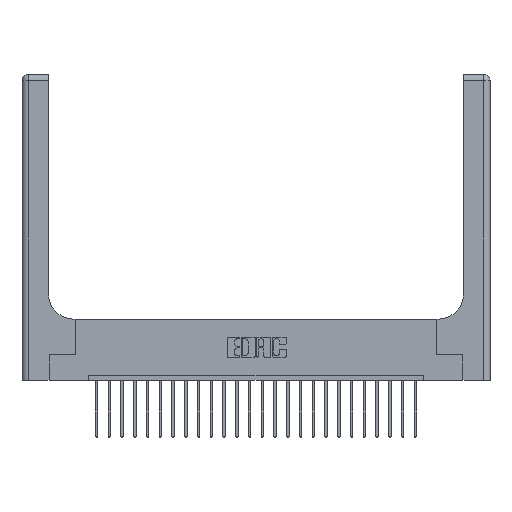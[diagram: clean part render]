
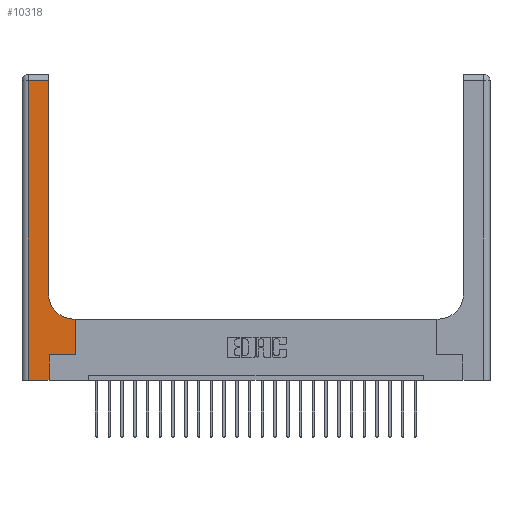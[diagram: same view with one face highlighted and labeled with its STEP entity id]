
A CAD part, top view. The second image highlights one B-rep face of the part: STEP entity #10318.
In plain terms, the highlighted planar face has unit normal (0, 0, 1).
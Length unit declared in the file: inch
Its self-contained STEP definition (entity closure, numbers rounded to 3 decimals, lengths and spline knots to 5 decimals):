
#536 = VERTEX_POINT ( 'NONE', #8447 ) ;
#696 = ORIENTED_EDGE ( 'NONE', *, *, #15866, .T. ) ;
#775 = VECTOR ( 'NONE', #949, 39.37008 ) ;
#890 = CARTESIAN_POINT ( 'NONE',  ( 0.51, 0.85, 0.37 ) ) ;
#949 = DIRECTION ( 'NONE',  ( 0., 1., 0. ) ) ;
#1411 = VECTOR ( 'NONE', #18639, 39.37008 ) ;
#1502 = CARTESIAN_POINT ( 'NONE',  ( 0.265, 0.25, 0.37 ) ) ;
#2010 = VERTEX_POINT ( 'NONE', #12377 ) ;
#2166 = EDGE_CURVE ( 'NONE', #536, #22480, #9101, .T. ) ;
#2348 = DIRECTION ( 'NONE',  ( 1., 0., 0. ) ) ;
#2523 = ORIENTED_EDGE ( 'NONE', *, *, #6751, .T. ) ;
#2749 = LINE ( 'NONE', #6005, #5046 ) ;
#3208 = FACE_OUTER_BOUND ( 'NONE', #9984, .T. ) ;
#3472 = DIRECTION ( 'NONE',  ( -1., 0., 0. ) ) ;
#3710 = ORIENTED_EDGE ( 'NONE', *, *, #13752, .T. ) ;
#3994 = CARTESIAN_POINT ( 'NONE',  ( 0.06, 2.94, 0.37 ) ) ;
#4312 = CARTESIAN_POINT ( 'NONE',  ( 0.265, 0.25, 0.37 ) ) ;
#4381 = LINE ( 'NONE', #12873, #12594 ) ;
#4400 = EDGE_CURVE ( 'NONE', #19987, #4777, #19600, .T. ) ;
#4777 = VERTEX_POINT ( 'NONE', #6236 ) ;
#5046 = VECTOR ( 'NONE', #22269, 39.37008 ) ;
#5268 = EDGE_CURVE ( 'NONE', #6876, #18994, #6587, .T. ) ;
#5833 = DIRECTION ( 'NONE',  ( 0., 0., -1. ) ) ;
#6005 = CARTESIAN_POINT ( 'NONE',  ( 0.528, 0.25, 0.37 ) ) ;
#6236 = CARTESIAN_POINT ( 'NONE',  ( 0.265, 0., 0.37 ) ) ;
#6587 = LINE ( 'NONE', #4312, #1411 ) ;
#6615 = VECTOR ( 'NONE', #22053, 39.37008 ) ;
#6751 = EDGE_CURVE ( 'NONE', #2010, #536, #17507, .T. ) ;
#6876 = VERTEX_POINT ( 'NONE', #1502 ) ;
#7293 = VERTEX_POINT ( 'NONE', #3994 ) ;
#7313 = EDGE_CURVE ( 'NONE', #18994, #2010, #2749, .T. ) ;
#7360 = DIRECTION ( 'NONE',  ( 0., -1., 0. ) ) ;
#7475 = VECTOR ( 'NONE', #3472, 39.37008 ) ;
#7632 = DIRECTION ( 'NONE',  ( -1., 0., 0. ) ) ;
#8279 = CARTESIAN_POINT ( 'NONE',  ( 0.265, 0., 0.37 ) ) ;
#8447 = CARTESIAN_POINT ( 'NONE',  ( 0.51, 0.6, 0.37 ) ) ;
#8545 = ORIENTED_EDGE ( 'NONE', *, *, #21210, .T. ) ;
#8591 = VECTOR ( 'NONE', #2348, 39.37008 ) ;
#8693 = DIRECTION ( 'NONE',  ( 0., 0., -1. ) ) ;
#9101 = CIRCLE ( 'NONE', #22188, 0.25 ) ;
#9984 = EDGE_LOOP ( 'NONE', ( #19673, #8545, #696, #13128, #3710, #21557, #15707, #2523, #17955 ) ) ;
#10123 = CARTESIAN_POINT ( 'NONE',  ( 0.26, 0.85, 0.37 ) ) ;
#10142 = LINE ( 'NONE', #8279, #775 ) ;
#10318 = ADVANCED_FACE ( 'NONE', ( #3208 ), #22109, .F. ) ;
#10768 = CARTESIAN_POINT ( 'NONE',  ( 0.26, 2.94, 0.37 ) ) ;
#10973 = CARTESIAN_POINT ( 'NONE',  ( 0.26, 3., 0.37 ) ) ;
#11373 = VERTEX_POINT ( 'NONE', #10768 ) ;
#11545 = EDGE_CURVE ( 'NONE', #22480, #11373, #21007, .T. ) ;
#11963 = AXIS2_PLACEMENT_3D ( 'NONE', #22193, #5833, #7632 ) ;
#12126 = VECTOR ( 'NONE', #15384, 39.37008 ) ;
#12369 = DIRECTION ( 'NONE',  ( 1., 0., 0. ) ) ;
#12377 = CARTESIAN_POINT ( 'NONE',  ( 0.528, 0.6, 0.37 ) ) ;
#12594 = VECTOR ( 'NONE', #7360, 39.37008 ) ;
#12873 = CARTESIAN_POINT ( 'NONE',  ( 0.06, 3., 0.37 ) ) ;
#13128 = ORIENTED_EDGE ( 'NONE', *, *, #4400, .T. ) ;
#13641 = CARTESIAN_POINT ( 'NONE',  ( 0.26, 0.6, 0.37 ) ) ;
#13752 = EDGE_CURVE ( 'NONE', #4777, #6876, #10142, .T. ) ;
#15004 = CARTESIAN_POINT ( 'NONE',  ( 0., 0., 0.37 ) ) ;
#15384 = DIRECTION ( 'NONE',  ( -1., 0., 0. ) ) ;
#15707 = ORIENTED_EDGE ( 'NONE', *, *, #7313, .T. ) ;
#15866 = EDGE_CURVE ( 'NONE', #7293, #19987, #4381, .T. ) ;
#15946 = CARTESIAN_POINT ( 'NONE',  ( 0.06, 0., 0.37 ) ) ;
#17507 = LINE ( 'NONE', #13641, #12126 ) ;
#17955 = ORIENTED_EDGE ( 'NONE', *, *, #2166, .T. ) ;
#18433 = CARTESIAN_POINT ( 'NONE',  ( 0., 2.94, 0.37 ) ) ;
#18639 = DIRECTION ( 'NONE',  ( 1., 0., 0. ) ) ;
#18994 = VERTEX_POINT ( 'NONE', #20430 ) ;
#19600 = LINE ( 'NONE', #15004, #8591 ) ;
#19673 = ORIENTED_EDGE ( 'NONE', *, *, #11545, .T. ) ;
#19987 = VERTEX_POINT ( 'NONE', #15946 ) ;
#20430 = CARTESIAN_POINT ( 'NONE',  ( 0.528, 0.25, 0.37 ) ) ;
#21007 = LINE ( 'NONE', #10973, #6615 ) ;
#21210 = EDGE_CURVE ( 'NONE', #11373, #7293, #22189, .T. ) ;
#21557 = ORIENTED_EDGE ( 'NONE', *, *, #5268, .T. ) ;
#22053 = DIRECTION ( 'NONE',  ( 0., 1., 0. ) ) ;
#22109 = PLANE ( 'NONE',  #11963 ) ;
#22188 = AXIS2_PLACEMENT_3D ( 'NONE', #890, #8693, #12369 ) ;
#22189 = LINE ( 'NONE', #18433, #7475 ) ;
#22193 = CARTESIAN_POINT ( 'NONE',  ( 0., 3., 0.37 ) ) ;
#22269 = DIRECTION ( 'NONE',  ( 0., 1., 0. ) ) ;
#22480 = VERTEX_POINT ( 'NONE', #10123 ) ;
